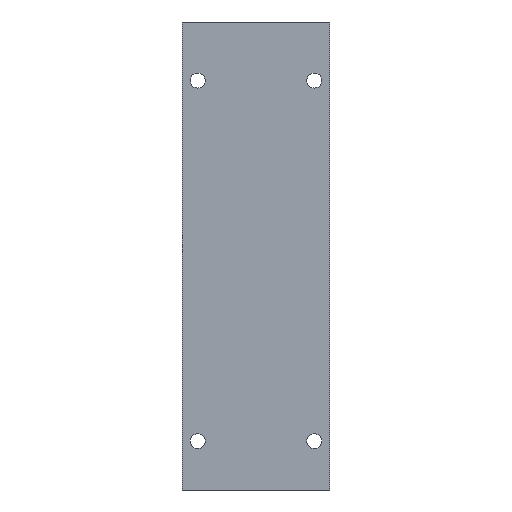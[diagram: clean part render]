
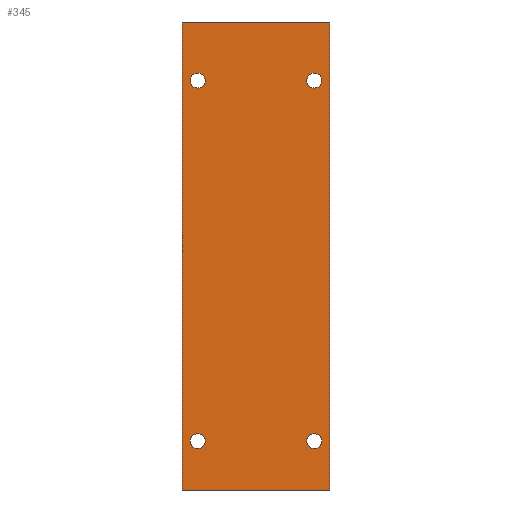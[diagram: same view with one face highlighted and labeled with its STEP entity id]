
A CAD part, left-side view. The second image highlights one B-rep face of the part: STEP entity #345.
In plain terms, the highlighted planar face has unit normal (-1, 0, 0).
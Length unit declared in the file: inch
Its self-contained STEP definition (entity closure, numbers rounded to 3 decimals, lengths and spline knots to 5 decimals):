
#15=FACE_BOUND('',#56,.T.);
#16=FACE_BOUND('',#57,.T.);
#17=FACE_BOUND('',#58,.T.);
#18=FACE_BOUND('',#59,.T.);
#23=PLANE('',#385);
#37=FACE_OUTER_BOUND('',#55,.T.);
#55=EDGE_LOOP('',(#253,#254,#255,#256));
#56=EDGE_LOOP('',(#257));
#57=EDGE_LOOP('',(#258));
#58=EDGE_LOOP('',(#259));
#59=EDGE_LOOP('',(#260));
#81=LINE('',#537,#113);
#82=LINE('',#539,#114);
#83=LINE('',#541,#115);
#84=LINE('',#542,#116);
#113=VECTOR('',#439,0.3937);
#114=VECTOR('',#440,0.3937);
#115=VECTOR('',#441,0.3937);
#116=VECTOR('',#442,0.3937);
#142=CIRCLE('',#375,0.0625);
#144=CIRCLE('',#378,0.0625);
#146=CIRCLE('',#381,0.0625);
#148=CIRCLE('',#384,0.0625);
#158=VERTEX_POINT('',#513);
#160=VERTEX_POINT('',#519);
#162=VERTEX_POINT('',#525);
#164=VERTEX_POINT('',#531);
#165=VERTEX_POINT('',#535);
#166=VERTEX_POINT('',#536);
#167=VERTEX_POINT('',#538);
#168=VERTEX_POINT('',#540);
#191=EDGE_CURVE('',#158,#158,#142,.T.);
#194=EDGE_CURVE('',#160,#160,#144,.T.);
#197=EDGE_CURVE('',#162,#162,#146,.T.);
#200=EDGE_CURVE('',#164,#164,#148,.T.);
#201=EDGE_CURVE('',#165,#166,#81,.T.);
#202=EDGE_CURVE('',#167,#165,#82,.T.);
#203=EDGE_CURVE('',#167,#168,#83,.T.);
#204=EDGE_CURVE('',#166,#168,#84,.T.);
#253=ORIENTED_EDGE('',*,*,#201,.F.);
#254=ORIENTED_EDGE('',*,*,#202,.F.);
#255=ORIENTED_EDGE('',*,*,#203,.T.);
#256=ORIENTED_EDGE('',*,*,#204,.F.);
#257=ORIENTED_EDGE('',*,*,#191,.T.);
#258=ORIENTED_EDGE('',*,*,#194,.T.);
#259=ORIENTED_EDGE('',*,*,#197,.T.);
#260=ORIENTED_EDGE('',*,*,#200,.T.);
#345=ADVANCED_FACE('',(#37,#15,#16,#17,#18),#23,.F.);
#375=AXIS2_PLACEMENT_3D('',#515,#414,#415);
#378=AXIS2_PLACEMENT_3D('',#521,#421,#422);
#381=AXIS2_PLACEMENT_3D('',#527,#428,#429);
#384=AXIS2_PLACEMENT_3D('',#533,#435,#436);
#385=AXIS2_PLACEMENT_3D('',#534,#437,#438);
#414=DIRECTION('center_axis',(1.,0.,0.));
#415=DIRECTION('ref_axis',(0.,0.,1.));
#421=DIRECTION('center_axis',(1.,0.,0.));
#422=DIRECTION('ref_axis',(0.,0.,1.));
#428=DIRECTION('center_axis',(1.,0.,0.));
#429=DIRECTION('ref_axis',(0.,0.,1.));
#435=DIRECTION('center_axis',(1.,0.,0.));
#436=DIRECTION('ref_axis',(0.,0.,1.));
#437=DIRECTION('center_axis',(1.,0.,0.));
#438=DIRECTION('ref_axis',(0.,0.,-1.));
#439=DIRECTION('',(0.,0.,1.));
#440=DIRECTION('',(0.,1.,0.));
#441=DIRECTION('',(0.,0.,1.));
#442=DIRECTION('',(0.,-1.,0.));
#513=CARTESIAN_POINT('',(-0.80475,0.10655,2.82523));
#515=CARTESIAN_POINT('Origin',(-0.80475,0.10655,2.88773));
#519=CARTESIAN_POINT('',(-0.80475,-0.87455,-0.20841));
#521=CARTESIAN_POINT('Origin',(-0.80475,-0.87455,-0.14591));
#525=CARTESIAN_POINT('',(-0.80475,-0.87455,2.82523));
#527=CARTESIAN_POINT('Origin',(-0.80475,-0.87455,2.88773));
#531=CARTESIAN_POINT('',(-0.80475,0.10655,-0.20841));
#533=CARTESIAN_POINT('Origin',(-0.80475,0.10655,-0.14591));
#534=CARTESIAN_POINT('Origin',(-0.80475,-0.384,1.41219));
#535=CARTESIAN_POINT('',(-0.80475,0.23622,-0.55631));
#536=CARTESIAN_POINT('',(-0.80475,0.23622,3.3807));
#537=CARTESIAN_POINT('',(-0.80475,0.23622,1.41219));
#538=CARTESIAN_POINT('',(-0.80475,-1.00422,-0.55631));
#539=CARTESIAN_POINT('',(-0.80475,-0.07389,-0.55631));
#540=CARTESIAN_POINT('',(-0.80475,-1.00422,3.3807));
#541=CARTESIAN_POINT('',(-0.80475,-1.00422,1.89644));
#542=CARTESIAN_POINT('',(-0.80475,-0.07389,3.3807));
